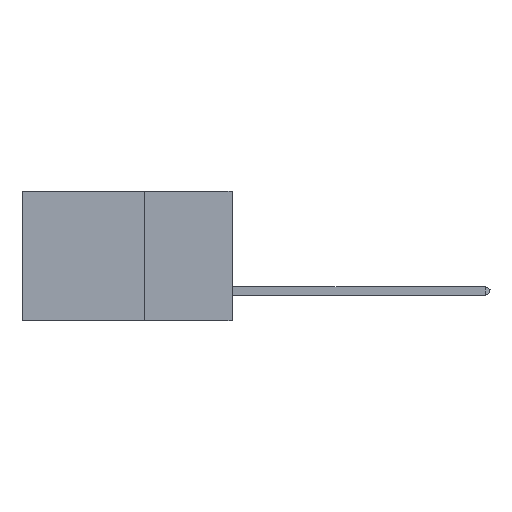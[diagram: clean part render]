
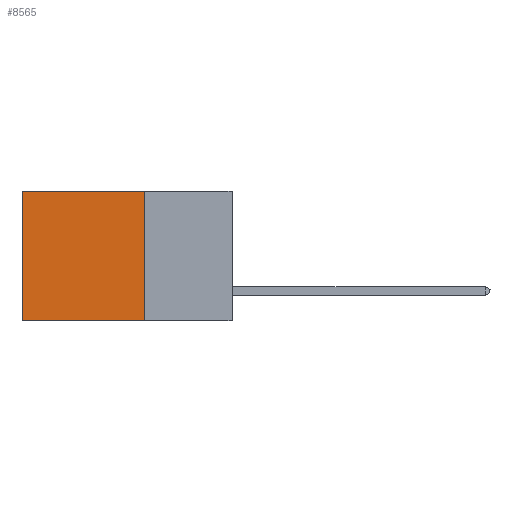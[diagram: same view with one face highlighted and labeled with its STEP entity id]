
A CAD part, left-side view. The second image highlights one B-rep face of the part: STEP entity #8565.
In plain terms, the highlighted planar face has unit normal (-1, 0, 0).
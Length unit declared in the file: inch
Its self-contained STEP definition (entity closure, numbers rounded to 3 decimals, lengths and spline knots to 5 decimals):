
#494 = VECTOR ( 'NONE', #23037, 39.37008 ) ;
#3704 = CARTESIAN_POINT ( 'NONE',  ( 0.2875, 0.25, 0. ) ) ;
#5387 = VECTOR ( 'NONE', #15803, 39.37008 ) ;
#6433 = ORIENTED_EDGE ( 'NONE', *, *, #21953, .F. ) ;
#6501 = FACE_OUTER_BOUND ( 'NONE', #28763, .T. ) ;
#7617 = EDGE_CURVE ( 'NONE', #20686, #25132, #26946, .T. ) ;
#8565 = ADVANCED_FACE ( 'NONE', ( #6501 ), #27804, .F. ) ;
#9086 = CARTESIAN_POINT ( 'NONE',  ( 0.2875, 0.25, -0.37 ) ) ;
#9475 = EDGE_CURVE ( 'NONE', #20686, #13559, #19533, .T. ) ;
#11725 = LINE ( 'NONE', #18139, #494 ) ;
#13090 = VECTOR ( 'NONE', #22796, 39.37008 ) ;
#13534 = VERTEX_POINT ( 'NONE', #25319 ) ;
#13559 = VERTEX_POINT ( 'NONE', #9086 ) ;
#14216 = EDGE_CURVE ( 'NONE', #25132, #13534, #19241, .T. ) ;
#14234 = ORIENTED_EDGE ( 'NONE', *, *, #9475, .F. ) ;
#14418 = CARTESIAN_POINT ( 'NONE',  ( 0.2875, 0.25, 0. ) ) ;
#15104 = CARTESIAN_POINT ( 'NONE',  ( 0.2875, 0.6, 0. ) ) ;
#15803 = DIRECTION ( 'NONE',  ( 0., 0., -1. ) ) ;
#16492 = DIRECTION ( 'NONE',  ( 1., 0., 0. ) ) ;
#16778 = DIRECTION ( 'NONE',  ( 0., 0., -1. ) ) ;
#18106 = CARTESIAN_POINT ( 'NONE',  ( 0.2875, 0.25, 0. ) ) ;
#18139 = CARTESIAN_POINT ( 'NONE',  ( 0.2875, 0.25, -0.37 ) ) ;
#18752 = CARTESIAN_POINT ( 'NONE',  ( 0.2875, 0.25, 0. ) ) ;
#19241 = LINE ( 'NONE', #25182, #5387 ) ;
#19533 = LINE ( 'NONE', #14418, #30111 ) ;
#20686 = VERTEX_POINT ( 'NONE', #3704 ) ;
#20894 = DIRECTION ( 'NONE',  ( 0., 0., -1. ) ) ;
#21953 = EDGE_CURVE ( 'NONE', #13559, #13534, #11725, .T. ) ;
#22796 = DIRECTION ( 'NONE',  ( 0., 1., 0. ) ) ;
#23037 = DIRECTION ( 'NONE',  ( 0., 1., 0. ) ) ;
#25132 = VERTEX_POINT ( 'NONE', #15104 ) ;
#25182 = CARTESIAN_POINT ( 'NONE',  ( 0.2875, 0.6, 0. ) ) ;
#25319 = CARTESIAN_POINT ( 'NONE',  ( 0.2875, 0.6, -0.37 ) ) ;
#26946 = LINE ( 'NONE', #18106, #13090 ) ;
#27667 = ORIENTED_EDGE ( 'NONE', *, *, #7617, .T. ) ;
#27804 = PLANE ( 'NONE',  #30004 ) ;
#28763 = EDGE_LOOP ( 'NONE', ( #29990, #6433, #14234, #27667 ) ) ;
#29990 = ORIENTED_EDGE ( 'NONE', *, *, #14216, .T. ) ;
#30004 = AXIS2_PLACEMENT_3D ( 'NONE', #18752, #16492, #20894 ) ;
#30111 = VECTOR ( 'NONE', #16778, 39.37008 ) ;
